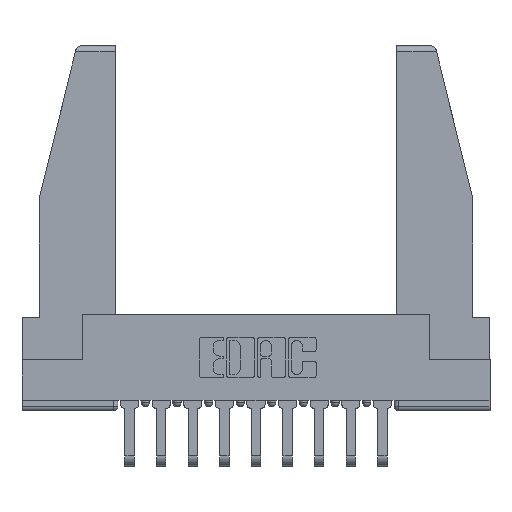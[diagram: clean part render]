
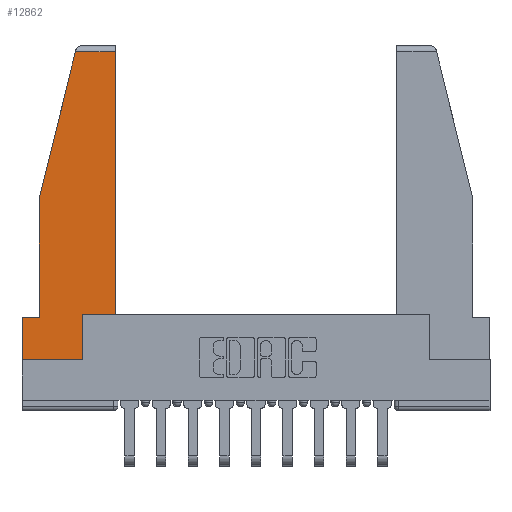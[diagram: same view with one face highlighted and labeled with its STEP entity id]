
A CAD part, top view. The second image highlights one B-rep face of the part: STEP entity #12862.
In plain terms, the highlighted planar face has unit normal (0, 0, 1).
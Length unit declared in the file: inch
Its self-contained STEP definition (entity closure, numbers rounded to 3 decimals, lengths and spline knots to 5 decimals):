
#360 = VERTEX_POINT ( 'NONE', #8579 ) ;
#437 = VERTEX_POINT ( 'NONE', #3134 ) ;
#638 = VECTOR ( 'NONE', #5222, 39.37008 ) ;
#785 = CARTESIAN_POINT ( 'NONE',  ( 0., 0., 0. ) ) ;
#859 = LINE ( 'NONE', #9552, #3465 ) ;
#956 = CARTESIAN_POINT ( 'NONE',  ( 0.271, 1.55, 0. ) ) ;
#962 = LINE ( 'NONE', #2318, #9846 ) ;
#987 = ORIENTED_EDGE ( 'NONE', *, *, #2353, .T. ) ;
#1185 = CARTESIAN_POINT ( 'NONE',  ( 0.086, 0.21, 0. ) ) ;
#1195 = ORIENTED_EDGE ( 'NONE', *, *, #2517, .T. ) ;
#1415 = EDGE_CURVE ( 'NONE', #437, #9716, #962, .T. ) ;
#2037 = CARTESIAN_POINT ( 'NONE',  ( 0.297, 0., 0. ) ) ;
#2054 = ORIENTED_EDGE ( 'NONE', *, *, #12229, .T. ) ;
#2064 = EDGE_LOOP ( 'NONE', ( #1195, #9247, #987, #2054, #7041, #2984, #8041, #5085, #3331 ) ) ;
#2170 = DIRECTION ( 'NONE',  ( 0., -1., 0. ) ) ;
#2211 = LINE ( 'NONE', #2037, #14328 ) ;
#2318 = CARTESIAN_POINT ( 'NONE',  ( 0.297, 0.223, 0. ) ) ;
#2353 = EDGE_CURVE ( 'NONE', #11853, #13737, #13431, .T. ) ;
#2517 = EDGE_CURVE ( 'NONE', #9716, #12195, #3364, .T. ) ;
#2640 = LINE ( 'NONE', #5531, #5223 ) ;
#2984 = ORIENTED_EDGE ( 'NONE', *, *, #7383, .T. ) ;
#3134 = CARTESIAN_POINT ( 'NONE',  ( 0.297, 0.223, 0. ) ) ;
#3193 = DIRECTION ( 'NONE',  ( 0., 1., 0. ) ) ;
#3254 = DIRECTION ( 'NONE',  ( 1., 0., 0. ) ) ;
#3317 = CARTESIAN_POINT ( 'NONE',  ( 0.086, 0.8, 0. ) ) ;
#3331 = ORIENTED_EDGE ( 'NONE', *, *, #1415, .T. ) ;
#3364 = LINE ( 'NONE', #5258, #14095 ) ;
#3465 = VECTOR ( 'NONE', #11822, 39.37008 ) ;
#3747 = CARTESIAN_POINT ( 'NONE',  ( 0.2636, 1.52, 0. ) ) ;
#4315 = PLANE ( 'NONE',  #7362 ) ;
#4859 = VERTEX_POINT ( 'NONE', #1185 ) ;
#5085 = ORIENTED_EDGE ( 'NONE', *, *, #8728, .T. ) ;
#5222 = DIRECTION ( 'NONE',  ( -1., 0., 0. ) ) ;
#5223 = VECTOR ( 'NONE', #12228, 39.37008 ) ;
#5258 = CARTESIAN_POINT ( 'NONE',  ( 0.461, 0.223, 0. ) ) ;
#5429 = LINE ( 'NONE', #5464, #7681 ) ;
#5464 = CARTESIAN_POINT ( 'NONE',  ( 0.086, 0.8, 0. ) ) ;
#5531 = CARTESIAN_POINT ( 'NONE',  ( 0., 0., 0. ) ) ;
#6799 = VECTOR ( 'NONE', #14111, 39.37008 ) ;
#7041 = ORIENTED_EDGE ( 'NONE', *, *, #8775, .T. ) ;
#7362 = AXIS2_PLACEMENT_3D ( 'NONE', #10068, #7721, #3254 ) ;
#7383 = EDGE_CURVE ( 'NONE', #9562, #9797, #859, .T. ) ;
#7681 = VECTOR ( 'NONE', #2170, 39.37008 ) ;
#7721 = DIRECTION ( 'NONE',  ( 0., 0., 1. ) ) ;
#8023 = FACE_OUTER_BOUND ( 'NONE', #2064, .T. ) ;
#8041 = ORIENTED_EDGE ( 'NONE', *, *, #12967, .T. ) ;
#8579 = CARTESIAN_POINT ( 'NONE',  ( 0.297, 0., 0. ) ) ;
#8728 = EDGE_CURVE ( 'NONE', #360, #437, #2211, .T. ) ;
#8775 = EDGE_CURVE ( 'NONE', #4859, #9562, #10718, .T. ) ;
#9019 = DIRECTION ( 'NONE',  ( 1., 0., 0. ) ) ;
#9247 = ORIENTED_EDGE ( 'NONE', *, *, #13625, .T. ) ;
#9552 = CARTESIAN_POINT ( 'NONE',  ( 0., 0.21, 0. ) ) ;
#9562 = VERTEX_POINT ( 'NONE', #12440 ) ;
#9650 = VECTOR ( 'NONE', #9855, 39.37008 ) ;
#9716 = VERTEX_POINT ( 'NONE', #14135 ) ;
#9797 = VERTEX_POINT ( 'NONE', #785 ) ;
#9846 = VECTOR ( 'NONE', #9019, 39.37008 ) ;
#9855 = DIRECTION ( 'NONE',  ( -0.239, -0.971, 0. ) ) ;
#10068 = CARTESIAN_POINT ( 'NONE',  ( 0., 0., 0. ) ) ;
#10718 = LINE ( 'NONE', #14126, #638 ) ;
#11822 = DIRECTION ( 'NONE',  ( 0., -1., 0. ) ) ;
#11853 = VERTEX_POINT ( 'NONE', #3747 ) ;
#12195 = VERTEX_POINT ( 'NONE', #13262 ) ;
#12228 = DIRECTION ( 'NONE',  ( 1., 0., 0. ) ) ;
#12229 = EDGE_CURVE ( 'NONE', #13737, #4859, #5429, .T. ) ;
#12440 = CARTESIAN_POINT ( 'NONE',  ( 0., 0.21, 0. ) ) ;
#12862 = ADVANCED_FACE ( 'NONE', ( #8023 ), #4315, .T. ) ;
#12967 = EDGE_CURVE ( 'NONE', #9797, #360, #2640, .T. ) ;
#13022 = DIRECTION ( 'NONE',  ( 0., 1., 0. ) ) ;
#13262 = CARTESIAN_POINT ( 'NONE',  ( 0.461, 1.52, 0. ) ) ;
#13385 = LINE ( 'NONE', #14005, #6799 ) ;
#13431 = LINE ( 'NONE', #956, #9650 ) ;
#13625 = EDGE_CURVE ( 'NONE', #12195, #11853, #13385, .T. ) ;
#13737 = VERTEX_POINT ( 'NONE', #3317 ) ;
#14005 = CARTESIAN_POINT ( 'NONE',  ( 0., 1.52, 0. ) ) ;
#14095 = VECTOR ( 'NONE', #13022, 39.37008 ) ;
#14111 = DIRECTION ( 'NONE',  ( -1., 0., 0. ) ) ;
#14126 = CARTESIAN_POINT ( 'NONE',  ( 0., 0.21, 0. ) ) ;
#14135 = CARTESIAN_POINT ( 'NONE',  ( 0.461, 0.223, 0. ) ) ;
#14328 = VECTOR ( 'NONE', #3193, 39.37008 ) ;
